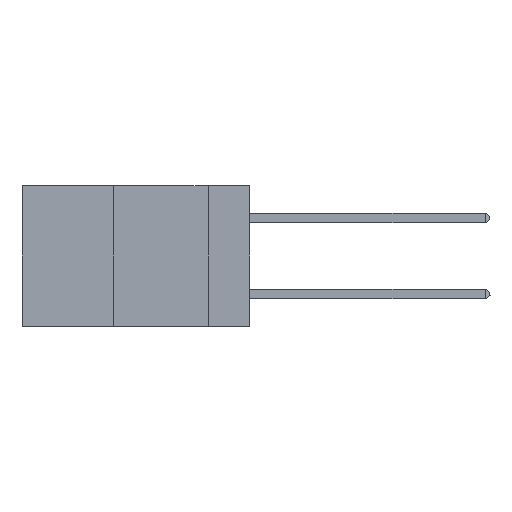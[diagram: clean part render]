
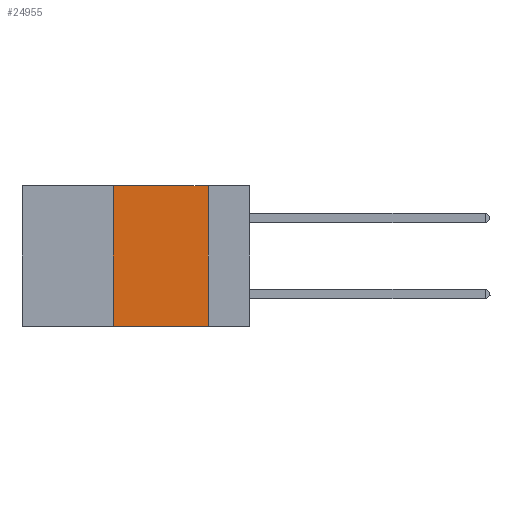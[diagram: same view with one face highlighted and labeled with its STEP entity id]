
A CAD part, left-side view. The second image highlights one B-rep face of the part: STEP entity #24955.
In plain terms, the highlighted planar face has unit normal (-1, 0, 0).
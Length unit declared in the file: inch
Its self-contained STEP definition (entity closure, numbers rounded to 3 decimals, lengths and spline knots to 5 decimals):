
#1041 = DIRECTION ( 'NONE',  ( 0., 0., -1. ) ) ;
#1304 = CARTESIAN_POINT ( 'NONE',  ( 0., 0.36, 0. ) ) ;
#1414 = CARTESIAN_POINT ( 'NONE',  ( 0., 0.6, 0. ) ) ;
#1465 = ORIENTED_EDGE ( 'NONE', *, *, #6629, .F. ) ;
#2007 = DIRECTION ( 'NONE',  ( 0., 0., 1. ) ) ;
#3021 = CARTESIAN_POINT ( 'NONE',  ( 0., 0.6, -0.37 ) ) ;
#3397 = DIRECTION ( 'NONE',  ( 0., -1., 0. ) ) ;
#3910 = EDGE_CURVE ( 'NONE', #7885, #9430, #14067, .T. ) ;
#5092 = CARTESIAN_POINT ( 'NONE',  ( 0., 0.36, 0. ) ) ;
#5306 = VECTOR ( 'NONE', #1041, 39.37008 ) ;
#5677 = VERTEX_POINT ( 'NONE', #19732 ) ;
#6629 = EDGE_CURVE ( 'NONE', #7885, #16650, #10239, .T. ) ;
#7373 = VECTOR ( 'NONE', #20616, 39.37008 ) ;
#7885 = VERTEX_POINT ( 'NONE', #19802 ) ;
#8631 = CARTESIAN_POINT ( 'NONE',  ( 0., 0.11, 0. ) ) ;
#8638 = CARTESIAN_POINT ( 'NONE',  ( 0., 0.6, 0. ) ) ;
#8722 = VECTOR ( 'NONE', #2007, 39.37008 ) ;
#8780 = ORIENTED_EDGE ( 'NONE', *, *, #12828, .F. ) ;
#9425 = LINE ( 'NONE', #1414, #16362 ) ;
#9430 = VERTEX_POINT ( 'NONE', #16116 ) ;
#10239 = LINE ( 'NONE', #5092, #8722 ) ;
#10619 = DIRECTION ( 'NONE',  ( 0., 0., -1. ) ) ;
#11971 = LINE ( 'NONE', #8631, #5306 ) ;
#12828 = EDGE_CURVE ( 'NONE', #5677, #9430, #11971, .T. ) ;
#14067 = LINE ( 'NONE', #3021, #7373 ) ;
#15304 = ORIENTED_EDGE ( 'NONE', *, *, #3910, .T. ) ;
#16116 = CARTESIAN_POINT ( 'NONE',  ( 0., 0.11, -0.37 ) ) ;
#16362 = VECTOR ( 'NONE', #3397, 39.37008 ) ;
#16650 = VERTEX_POINT ( 'NONE', #1304 ) ;
#17481 = FACE_OUTER_BOUND ( 'NONE', #19095, .T. ) ;
#17778 = AXIS2_PLACEMENT_3D ( 'NONE', #8638, #18550, #10619 ) ;
#18550 = DIRECTION ( 'NONE',  ( 1., 0., 0. ) ) ;
#19095 = EDGE_LOOP ( 'NONE', ( #8780, #23032, #1465, #15304 ) ) ;
#19732 = CARTESIAN_POINT ( 'NONE',  ( 0., 0.11, 0. ) ) ;
#19802 = CARTESIAN_POINT ( 'NONE',  ( 0., 0.36, -0.37 ) ) ;
#20351 = PLANE ( 'NONE',  #17778 ) ;
#20616 = DIRECTION ( 'NONE',  ( 0., -1., 0. ) ) ;
#22697 = EDGE_CURVE ( 'NONE', #16650, #5677, #9425, .T. ) ;
#23032 = ORIENTED_EDGE ( 'NONE', *, *, #22697, .F. ) ;
#24955 = ADVANCED_FACE ( 'NONE', ( #17481 ), #20351, .F. ) ;
